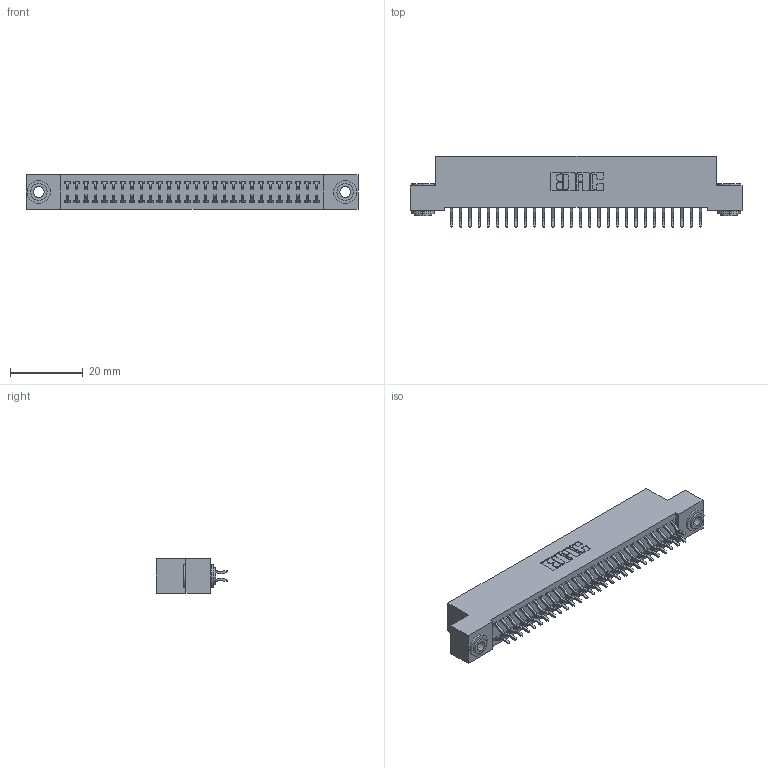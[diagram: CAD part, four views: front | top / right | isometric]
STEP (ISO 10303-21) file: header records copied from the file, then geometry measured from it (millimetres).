
FILE_DESCRIPTION (( 'STEP AP203' ), '1' );
FILE_NAME ('392-056-556-203.STEP', '2019-10-08T15:26:09', ( '' ), ( '' ), 'SwSTEP 2.0', 'SolidWorks 2016', '' );
FILE_SCHEMA (( 'CONFIG_CONTROL_DESIGN' ));
Length unit declared in the file: inch
Products named in the file (4): 342 Part_.156 TH; 345-292-001_556 Tail; 342-250-002_345-250-002-102; 392-056-556-203
Assembly tree (59 placements, depth 2):
  392-056-556-203
    342 Part_.156 TH
    345-292-001_556 Tail  x56
    342-250-002_345-250-002-102  x2
Bounding box: 91.44 x 19.58 x 9.4 mm (x, y, z)
Volume: 8171 mm3; surface area: 13115.1 mm2
Topology: 59 solids, 59 shells, 3396 faces, 10063 edges, 6630 vertices
Faces by surface type: plane 2316, cylinder 1072, cone 8
Entity records: 20562 total; most frequent: CARTESIAN_POINT 3413, ORIENTED_EDGE 3330, DIRECTION 2963, EDGE_CURVE 1665, VECTOR 1505, LINE 1505, VERTEX_POINT 1106, AXIS2_PLACEMENT_3D 729
